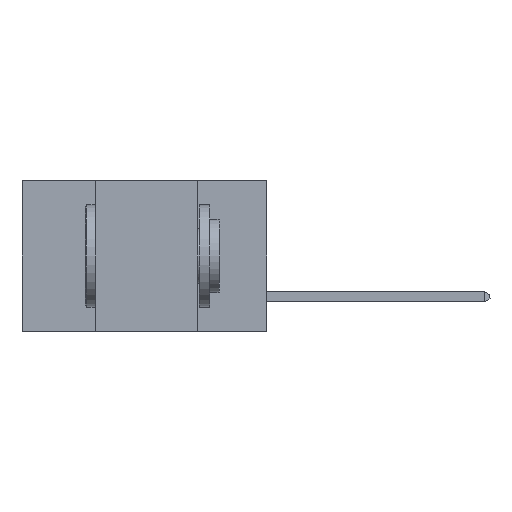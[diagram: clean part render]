
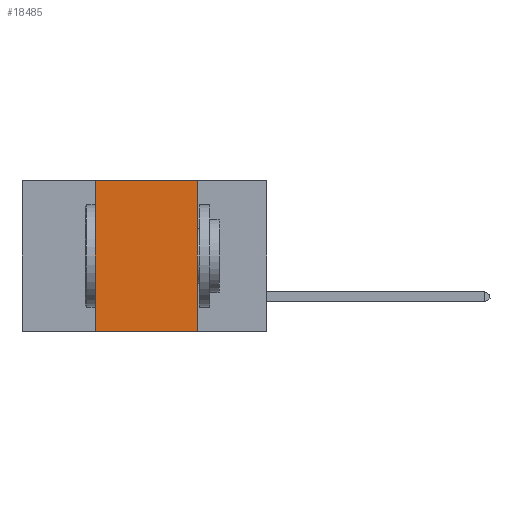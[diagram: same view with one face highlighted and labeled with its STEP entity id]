
A CAD part, left-side view. The second image highlights one B-rep face of the part: STEP entity #18485.
In plain terms, the highlighted planar face has unit normal (-1, 0, 0).
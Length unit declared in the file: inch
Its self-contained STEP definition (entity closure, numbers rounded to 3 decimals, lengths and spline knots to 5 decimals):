
#2276 = EDGE_LOOP ( 'NONE', ( #15846, #19253, #3625, #25549 ) ) ;
#3446 = CARTESIAN_POINT ( 'NONE',  ( 0., 0.6, -0.37 ) ) ;
#3577 = VECTOR ( 'NONE', #22524, 39.37008 ) ;
#3625 = ORIENTED_EDGE ( 'NONE', *, *, #7252, .F. ) ;
#4245 = CARTESIAN_POINT ( 'NONE',  ( 0., 0.17, 0. ) ) ;
#4869 = PLANE ( 'NONE',  #21409 ) ;
#5323 = CARTESIAN_POINT ( 'NONE',  ( 0., 0.42, 0. ) ) ;
#5889 = CARTESIAN_POINT ( 'NONE',  ( 0., 0.42, 0. ) ) ;
#7252 = EDGE_CURVE ( 'NONE', #25553, #12941, #18393, .T. ) ;
#8837 = LINE ( 'NONE', #3446, #17055 ) ;
#9546 = DIRECTION ( 'NONE',  ( 0., -1., 0. ) ) ;
#10343 = CARTESIAN_POINT ( 'NONE',  ( 0., 0.6, 0. ) ) ;
#12173 = LINE ( 'NONE', #32816, #32571 ) ;
#12941 = VERTEX_POINT ( 'NONE', #5323 ) ;
#13256 = DIRECTION ( 'NONE',  ( 1., 0., 0. ) ) ;
#13386 = DIRECTION ( 'NONE',  ( 0., 0., -1. ) ) ;
#13852 = VECTOR ( 'NONE', #9546, 39.37008 ) ;
#15846 = ORIENTED_EDGE ( 'NONE', *, *, #33981, .F. ) ;
#16888 = CARTESIAN_POINT ( 'NONE',  ( 0., 0.17, -0.37 ) ) ;
#17055 = VECTOR ( 'NONE', #22957, 39.37008 ) ;
#17848 = CARTESIAN_POINT ( 'NONE',  ( 0., 0.42, -0.37 ) ) ;
#18393 = LINE ( 'NONE', #5889, #3577 ) ;
#18485 = ADVANCED_FACE ( 'NONE', ( #24858 ), #4869, .F. ) ;
#19253 = ORIENTED_EDGE ( 'NONE', *, *, #29196, .F. ) ;
#20593 = CARTESIAN_POINT ( 'NONE',  ( 0., 0.6, 0. ) ) ;
#21236 = LINE ( 'NONE', #20593, #13852 ) ;
#21409 = AXIS2_PLACEMENT_3D ( 'NONE', #10343, #13256, #32690 ) ;
#21588 = VERTEX_POINT ( 'NONE', #16888 ) ;
#22524 = DIRECTION ( 'NONE',  ( 0., 0., 1. ) ) ;
#22957 = DIRECTION ( 'NONE',  ( 0., -1., 0. ) ) ;
#24858 = FACE_OUTER_BOUND ( 'NONE', #2276, .T. ) ;
#25549 = ORIENTED_EDGE ( 'NONE', *, *, #26576, .T. ) ;
#25553 = VERTEX_POINT ( 'NONE', #17848 ) ;
#26576 = EDGE_CURVE ( 'NONE', #25553, #21588, #8837, .T. ) ;
#29196 = EDGE_CURVE ( 'NONE', #12941, #33770, #21236, .T. ) ;
#32571 = VECTOR ( 'NONE', #13386, 39.37008 ) ;
#32690 = DIRECTION ( 'NONE',  ( 0., 0., -1. ) ) ;
#32816 = CARTESIAN_POINT ( 'NONE',  ( 0., 0.17, 0. ) ) ;
#33770 = VERTEX_POINT ( 'NONE', #4245 ) ;
#33981 = EDGE_CURVE ( 'NONE', #33770, #21588, #12173, .T. ) ;
